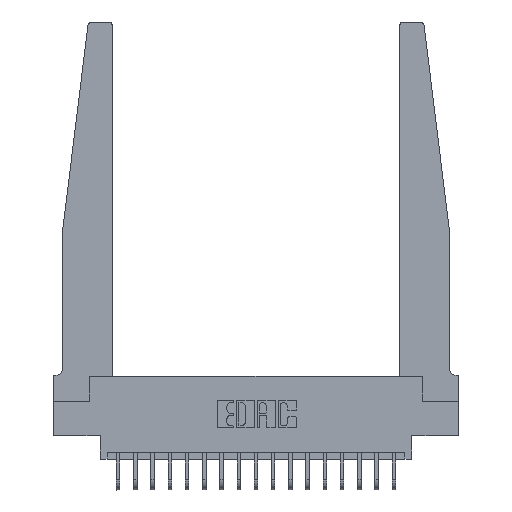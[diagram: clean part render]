
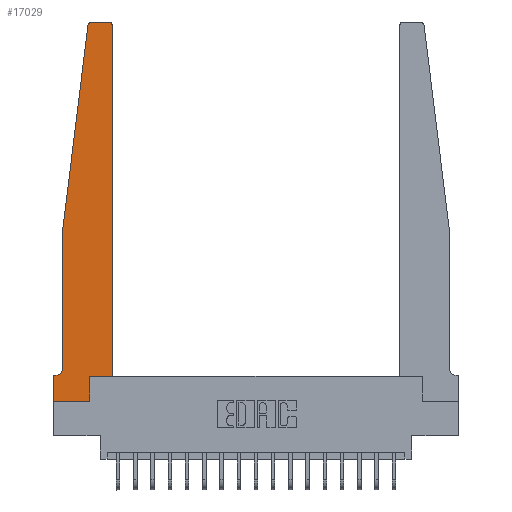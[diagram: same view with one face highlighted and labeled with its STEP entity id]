
A CAD part, top view. The second image highlights one B-rep face of the part: STEP entity #17029.
In plain terms, the highlighted planar face has unit normal (0, 0, 1).
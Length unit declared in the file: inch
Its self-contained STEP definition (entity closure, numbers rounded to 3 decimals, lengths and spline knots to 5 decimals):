
#110 = VERTEX_POINT ( 'NONE', #15070 ) ;
#138 = EDGE_CURVE ( 'NONE', #19190, #16808, #19370, .T. ) ;
#522 = EDGE_LOOP ( 'NONE', ( #3055, #14550, #14489, #16378, #5330, #20044, #19466, #7630, #20197, #10369, #9318, #2216 ) ) ;
#553 = DIRECTION ( 'NONE',  ( 0., 0., 1. ) ) ;
#1094 = VERTEX_POINT ( 'NONE', #15197 ) ;
#1838 = DIRECTION ( 'NONE',  ( 1., 0., 0. ) ) ;
#2135 = DIRECTION ( 'NONE',  ( 0., 1., 0. ) ) ;
#2216 = ORIENTED_EDGE ( 'NONE', *, *, #19378, .T. ) ;
#3055 = ORIENTED_EDGE ( 'NONE', *, *, #8677, .T. ) ;
#3285 = VERTEX_POINT ( 'NONE', #20760 ) ;
#3772 = DIRECTION ( 'NONE',  ( 1., 0., 0. ) ) ;
#4028 = LINE ( 'NONE', #9218, #16514 ) ;
#4233 = EDGE_CURVE ( 'NONE', #6931, #13111, #17398, .T. ) ;
#4330 = CARTESIAN_POINT ( 'NONE',  ( 0.015, 0.2375, 0.37 ) ) ;
#4585 = CARTESIAN_POINT ( 'NONE',  ( 0.065, 1.25, 0.37 ) ) ;
#4655 = EDGE_CURVE ( 'NONE', #6826, #12863, #7137, .T. ) ;
#4786 = CARTESIAN_POINT ( 'NONE',  ( 0., 0., 0.37 ) ) ;
#5201 = CARTESIAN_POINT ( 'NONE',  ( 0.425, 0.18, 0.37 ) ) ;
#5282 = VERTEX_POINT ( 'NONE', #5452 ) ;
#5330 = ORIENTED_EDGE ( 'NONE', *, *, #7721, .T. ) ;
#5452 = CARTESIAN_POINT ( 'NONE',  ( 0.24675, 2.72367, 0.37 ) ) ;
#5853 = EDGE_CURVE ( 'NONE', #110, #6826, #20682, .T. ) ;
#6383 = LINE ( 'NONE', #7135, #18154 ) ;
#6826 = VERTEX_POINT ( 'NONE', #12784 ) ;
#6931 = VERTEX_POINT ( 'NONE', #11400 ) ;
#7121 = EDGE_CURVE ( 'NONE', #13111, #12088, #6383, .T. ) ;
#7135 = CARTESIAN_POINT ( 'NONE',  ( 0.425, 0.18, 0.37 ) ) ;
#7137 = LINE ( 'NONE', #4786, #11700 ) ;
#7166 = CARTESIAN_POINT ( 'NONE',  ( 0., 0.1875, 0.37 ) ) ;
#7268 = DIRECTION ( 'NONE',  ( 0., 1., 0. ) ) ;
#7327 = EDGE_CURVE ( 'NONE', #5282, #19190, #10700, .T. ) ;
#7630 = ORIENTED_EDGE ( 'NONE', *, *, #17206, .T. ) ;
#7721 = EDGE_CURVE ( 'NONE', #16808, #110, #19406, .T. ) ;
#7726 = AXIS2_PLACEMENT_3D ( 'NONE', #8521, #8323, #3772 ) ;
#8074 = EDGE_CURVE ( 'NONE', #3285, #5282, #17610, .T. ) ;
#8323 = DIRECTION ( 'NONE',  ( 0., 0., 1. ) ) ;
#8521 = CARTESIAN_POINT ( 'NONE',  ( 0.395, 2.72, 0.37 ) ) ;
#8677 = EDGE_CURVE ( 'NONE', #1094, #3285, #12933, .T. ) ;
#8679 = VECTOR ( 'NONE', #7268, 39.37008 ) ;
#8751 = DIRECTION ( 'NONE',  ( 1., 0., 0. ) ) ;
#8848 = VECTOR ( 'NONE', #13371, 39.37008 ) ;
#8893 = CARTESIAN_POINT ( 'NONE',  ( 0.2605, 0.18, 0.37 ) ) ;
#8916 = VECTOR ( 'NONE', #9325, 39.37008 ) ;
#9218 = CARTESIAN_POINT ( 'NONE',  ( 0., 0., 0.37 ) ) ;
#9318 = ORIENTED_EDGE ( 'NONE', *, *, #9366, .T. ) ;
#9325 = DIRECTION ( 'NONE',  ( -0.122, -0.992, 0. ) ) ;
#9366 = EDGE_CURVE ( 'NONE', #12088, #12702, #17282, .T. ) ;
#9972 = CARTESIAN_POINT ( 'NONE',  ( 0.25, 2.75, 0.37 ) ) ;
#10369 = ORIENTED_EDGE ( 'NONE', *, *, #7121, .T. ) ;
#10700 = LINE ( 'NONE', #4585, #8916 ) ;
#11066 = CARTESIAN_POINT ( 'NONE',  ( 0.065, 1.25, 0.37 ) ) ;
#11386 = VECTOR ( 'NONE', #18339, 39.37008 ) ;
#11400 = CARTESIAN_POINT ( 'NONE',  ( 0.2605, 0., 0.37 ) ) ;
#11608 = VECTOR ( 'NONE', #2135, 39.37008 ) ;
#11700 = VECTOR ( 'NONE', #19553, 39.37008 ) ;
#11897 = FACE_OUTER_BOUND ( 'NONE', #522, .T. ) ;
#12088 = VERTEX_POINT ( 'NONE', #5201 ) ;
#12125 = CARTESIAN_POINT ( 'NONE',  ( 0., 0., 0.37 ) ) ;
#12475 = VECTOR ( 'NONE', #13576, 39.37008 ) ;
#12702 = VERTEX_POINT ( 'NONE', #16492 ) ;
#12784 = CARTESIAN_POINT ( 'NONE',  ( 0., 0.1875, 0.37 ) ) ;
#12838 = CARTESIAN_POINT ( 'NONE',  ( 0.2605, 0.18, 0.37 ) ) ;
#12863 = VERTEX_POINT ( 'NONE', #12125 ) ;
#12933 = LINE ( 'NONE', #9972, #8848 ) ;
#13111 = VERTEX_POINT ( 'NONE', #12838 ) ;
#13366 = CARTESIAN_POINT ( 'NONE',  ( 0.065, 0.1875, 0.37 ) ) ;
#13371 = DIRECTION ( 'NONE',  ( -1., 0., 0. ) ) ;
#13487 = CARTESIAN_POINT ( 'NONE',  ( 0.065, 1.25, 0.37 ) ) ;
#13576 = DIRECTION ( 'NONE',  ( -1., 0., 0. ) ) ;
#13624 = PLANE ( 'NONE',  #16024 ) ;
#14489 = ORIENTED_EDGE ( 'NONE', *, *, #7327, .T. ) ;
#14550 = ORIENTED_EDGE ( 'NONE', *, *, #8074, .T. ) ;
#15070 = CARTESIAN_POINT ( 'NONE',  ( 0.015, 0.1875, 0.37 ) ) ;
#15197 = CARTESIAN_POINT ( 'NONE',  ( 0.395, 2.75, 0.37 ) ) ;
#15277 = DIRECTION ( 'NONE',  ( 1., 0., 0. ) ) ;
#15358 = AXIS2_PLACEMENT_3D ( 'NONE', #4330, #17465, #15706 ) ;
#15381 = CIRCLE ( 'NONE', #7726, 0.03 ) ;
#15706 = DIRECTION ( 'NONE',  ( -1., 0., 0. ) ) ;
#16024 = AXIS2_PLACEMENT_3D ( 'NONE', #7166, #553, #15277 ) ;
#16378 = ORIENTED_EDGE ( 'NONE', *, *, #138, .T. ) ;
#16492 = CARTESIAN_POINT ( 'NONE',  ( 0.425, 2.72, 0.37 ) ) ;
#16514 = VECTOR ( 'NONE', #20666, 39.37008 ) ;
#16722 = CARTESIAN_POINT ( 'NONE',  ( 0.425, 0.18, 0.37 ) ) ;
#16808 = VERTEX_POINT ( 'NONE', #17832 ) ;
#17029 = ADVANCED_FACE ( 'NONE', ( #11897 ), #13624, .T. ) ;
#17206 = EDGE_CURVE ( 'NONE', #12863, #6931, #4028, .T. ) ;
#17282 = LINE ( 'NONE', #16722, #11608 ) ;
#17398 = LINE ( 'NONE', #8893, #8679 ) ;
#17465 = DIRECTION ( 'NONE',  ( 0., 0., -1. ) ) ;
#17610 = CIRCLE ( 'NONE', #20585, 0.03 ) ;
#17832 = CARTESIAN_POINT ( 'NONE',  ( 0.065, 0.2375, 0.37 ) ) ;
#18154 = VECTOR ( 'NONE', #8751, 39.37008 ) ;
#18339 = DIRECTION ( 'NONE',  ( 0., -1., 0. ) ) ;
#19190 = VERTEX_POINT ( 'NONE', #11066 ) ;
#19370 = LINE ( 'NONE', #13487, #11386 ) ;
#19378 = EDGE_CURVE ( 'NONE', #12702, #1094, #15381, .T. ) ;
#19406 = CIRCLE ( 'NONE', #15358, 0.05 ) ;
#19466 = ORIENTED_EDGE ( 'NONE', *, *, #4655, .T. ) ;
#19553 = DIRECTION ( 'NONE',  ( 0., -1., 0. ) ) ;
#19662 = DIRECTION ( 'NONE',  ( 0., 0., 1. ) ) ;
#19728 = CARTESIAN_POINT ( 'NONE',  ( 0.27653, 2.72, 0.37 ) ) ;
#20044 = ORIENTED_EDGE ( 'NONE', *, *, #5853, .T. ) ;
#20197 = ORIENTED_EDGE ( 'NONE', *, *, #4233, .T. ) ;
#20585 = AXIS2_PLACEMENT_3D ( 'NONE', #19728, #19662, #1838 ) ;
#20666 = DIRECTION ( 'NONE',  ( 1., 0., 0. ) ) ;
#20682 = LINE ( 'NONE', #13366, #12475 ) ;
#20760 = CARTESIAN_POINT ( 'NONE',  ( 0.27653, 2.75, 0.37 ) ) ;
